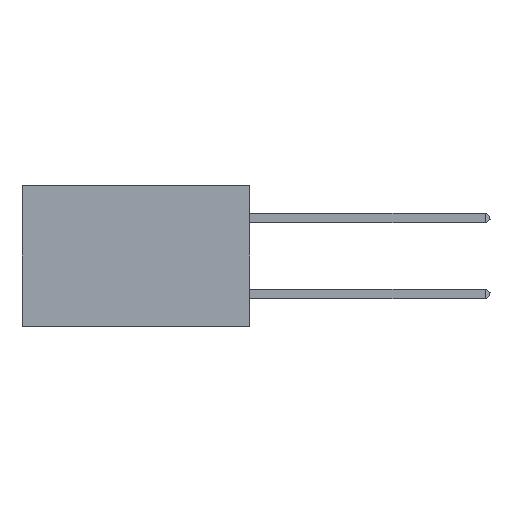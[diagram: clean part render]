
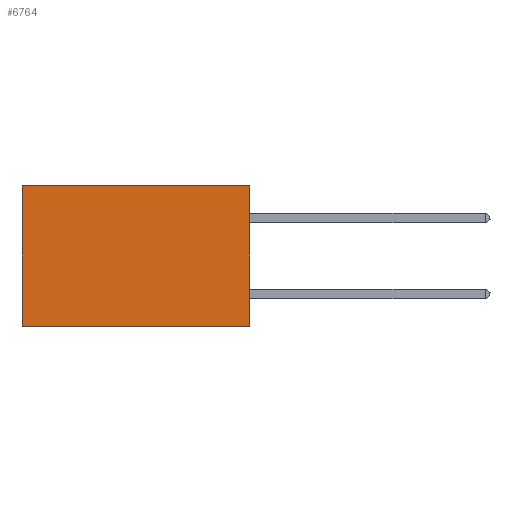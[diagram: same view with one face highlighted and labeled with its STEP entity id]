
A CAD part, left-side view. The second image highlights one B-rep face of the part: STEP entity #6764.
In plain terms, the highlighted planar face has unit normal (-1, 0, 0).
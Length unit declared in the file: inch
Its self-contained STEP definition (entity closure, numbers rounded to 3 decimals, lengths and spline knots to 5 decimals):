
#273 = CARTESIAN_POINT ( 'NONE',  ( 0.2875, 0., 0. ) ) ;
#316 = ORIENTED_EDGE ( 'NONE', *, *, #4218, .T. ) ;
#409 = VERTEX_POINT ( 'NONE', #9997 ) ;
#593 = VECTOR ( 'NONE', #16609, 39.37008 ) ;
#1485 = DIRECTION ( 'NONE',  ( 0., 0., -1. ) ) ;
#2289 = LINE ( 'NONE', #13331, #13679 ) ;
#2576 = VERTEX_POINT ( 'NONE', #15049 ) ;
#3701 = DIRECTION ( 'NONE',  ( 1., 0., 0. ) ) ;
#3991 = CARTESIAN_POINT ( 'NONE',  ( 0.2875, 0., -0.37 ) ) ;
#4218 = EDGE_CURVE ( 'NONE', #2576, #409, #2289, .T. ) ;
#4321 = DIRECTION ( 'NONE',  ( 0., 0., -1. ) ) ;
#4617 = EDGE_CURVE ( 'NONE', #4952, #18976, #16292, .T. ) ;
#4952 = VERTEX_POINT ( 'NONE', #17568 ) ;
#5981 = EDGE_CURVE ( 'NONE', #409, #18976, #11198, .T. ) ;
#6490 = CARTESIAN_POINT ( 'NONE',  ( 0.2875, 0.6, 0. ) ) ;
#6702 = ORIENTED_EDGE ( 'NONE', *, *, #7561, .F. ) ;
#6764 = ADVANCED_FACE ( 'NONE', ( #7538 ), #10416, .F. ) ;
#7538 = FACE_OUTER_BOUND ( 'NONE', #9873, .T. ) ;
#7561 = EDGE_CURVE ( 'NONE', #2576, #4952, #9368, .T. ) ;
#7836 = VECTOR ( 'NONE', #12137, 39.37008 ) ;
#9368 = LINE ( 'NONE', #273, #593 ) ;
#9873 = EDGE_LOOP ( 'NONE', ( #16568, #16288, #6702, #316 ) ) ;
#9997 = CARTESIAN_POINT ( 'NONE',  ( 0.2875, 0.6, 0. ) ) ;
#10416 = PLANE ( 'NONE',  #15794 ) ;
#10754 = VECTOR ( 'NONE', #4321, 39.37008 ) ;
#11198 = LINE ( 'NONE', #6490, #10754 ) ;
#12137 = DIRECTION ( 'NONE',  ( 0., 1., 0. ) ) ;
#12924 = DIRECTION ( 'NONE',  ( 0., 1., 0. ) ) ;
#13331 = CARTESIAN_POINT ( 'NONE',  ( 0.2875, 0., 0. ) ) ;
#13679 = VECTOR ( 'NONE', #12924, 39.37008 ) ;
#15049 = CARTESIAN_POINT ( 'NONE',  ( 0.2875, 0., 0. ) ) ;
#15794 = AXIS2_PLACEMENT_3D ( 'NONE', #18789, #3701, #1485 ) ;
#16288 = ORIENTED_EDGE ( 'NONE', *, *, #4617, .F. ) ;
#16292 = LINE ( 'NONE', #3991, #7836 ) ;
#16568 = ORIENTED_EDGE ( 'NONE', *, *, #5981, .T. ) ;
#16609 = DIRECTION ( 'NONE',  ( 0., 0., -1. ) ) ;
#17568 = CARTESIAN_POINT ( 'NONE',  ( 0.2875, 0., -0.37 ) ) ;
#18202 = CARTESIAN_POINT ( 'NONE',  ( 0.2875, 0.6, -0.37 ) ) ;
#18789 = CARTESIAN_POINT ( 'NONE',  ( 0.2875, 0., 0. ) ) ;
#18976 = VERTEX_POINT ( 'NONE', #18202 ) ;
